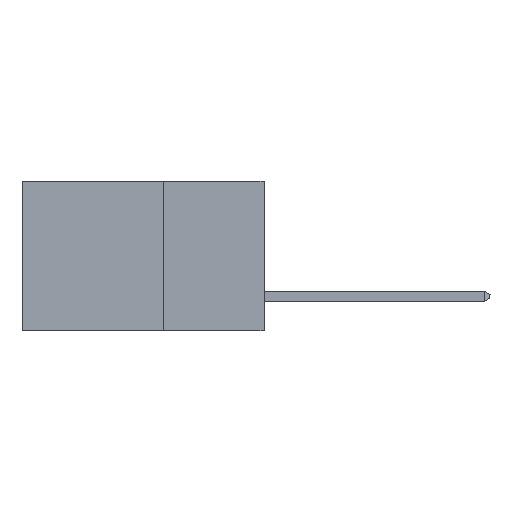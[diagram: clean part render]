
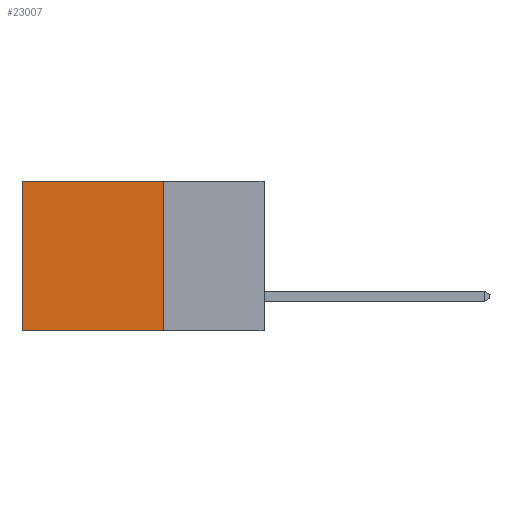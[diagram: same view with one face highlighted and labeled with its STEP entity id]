
A CAD part, left-side view. The second image highlights one B-rep face of the part: STEP entity #23007.
In plain terms, the highlighted planar face has unit normal (-1, 0, 0).
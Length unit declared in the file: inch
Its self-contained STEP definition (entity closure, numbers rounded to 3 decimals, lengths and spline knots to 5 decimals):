
#675 = ORIENTED_EDGE ( 'NONE', *, *, #10775, .F. ) ;
#1658 = LINE ( 'NONE', #20519, #21011 ) ;
#4013 = LINE ( 'NONE', #20035, #21431 ) ;
#5081 = CARTESIAN_POINT ( 'NONE',  ( 0.298, 0.25, 0. ) ) ;
#5566 = DIRECTION ( 'NONE',  ( 0., 0., -1. ) ) ;
#6432 = VERTEX_POINT ( 'NONE', #14253 ) ;
#7461 = ORIENTED_EDGE ( 'NONE', *, *, #23167, .F. ) ;
#7675 = EDGE_CURVE ( 'NONE', #17527, #6432, #8095, .T. ) ;
#7882 = DIRECTION ( 'NONE',  ( 0., 0., -1. ) ) ;
#8093 = FACE_OUTER_BOUND ( 'NONE', #15629, .T. ) ;
#8095 = LINE ( 'NONE', #14112, #16830 ) ;
#10775 = EDGE_CURVE ( 'NONE', #18205, #21347, #20278, .T. ) ;
#10974 = CARTESIAN_POINT ( 'NONE',  ( 0.298, 0.6, -0.37 ) ) ;
#12335 = ORIENTED_EDGE ( 'NONE', *, *, #7675, .T. ) ;
#12985 = DIRECTION ( 'NONE',  ( 0., 0., -1. ) ) ;
#13884 = CARTESIAN_POINT ( 'NONE',  ( 0.298, 0.25, -0.37 ) ) ;
#14112 = CARTESIAN_POINT ( 'NONE',  ( 0.298, 0.25, 0. ) ) ;
#14253 = CARTESIAN_POINT ( 'NONE',  ( 0.298, 0.6, 0. ) ) ;
#14507 = CARTESIAN_POINT ( 'NONE',  ( 0.298, 0.25, 0. ) ) ;
#14585 = PLANE ( 'NONE',  #20897 ) ;
#15629 = EDGE_LOOP ( 'NONE', ( #18338, #675, #7461, #12335 ) ) ;
#16830 = VECTOR ( 'NONE', #17787, 39.37008 ) ;
#17527 = VERTEX_POINT ( 'NONE', #5081 ) ;
#17787 = DIRECTION ( 'NONE',  ( 0., 1., 0. ) ) ;
#18205 = VERTEX_POINT ( 'NONE', #20678 ) ;
#18338 = ORIENTED_EDGE ( 'NONE', *, *, #20608, .T. ) ;
#20035 = CARTESIAN_POINT ( 'NONE',  ( 0.298, 0.6, 0. ) ) ;
#20278 = LINE ( 'NONE', #13884, #22532 ) ;
#20401 = DIRECTION ( 'NONE',  ( 0., 1., 0. ) ) ;
#20519 = CARTESIAN_POINT ( 'NONE',  ( 0.298, 0.25, 0. ) ) ;
#20608 = EDGE_CURVE ( 'NONE', #6432, #21347, #4013, .T. ) ;
#20678 = CARTESIAN_POINT ( 'NONE',  ( 0.298, 0.25, -0.37 ) ) ;
#20897 = AXIS2_PLACEMENT_3D ( 'NONE', #14507, #21709, #5566 ) ;
#21011 = VECTOR ( 'NONE', #7882, 39.37008 ) ;
#21347 = VERTEX_POINT ( 'NONE', #10974 ) ;
#21431 = VECTOR ( 'NONE', #12985, 39.37008 ) ;
#21709 = DIRECTION ( 'NONE',  ( 1., 0., 0. ) ) ;
#22532 = VECTOR ( 'NONE', #20401, 39.37008 ) ;
#23007 = ADVANCED_FACE ( 'NONE', ( #8093 ), #14585, .F. ) ;
#23167 = EDGE_CURVE ( 'NONE', #17527, #18205, #1658, .T. ) ;
